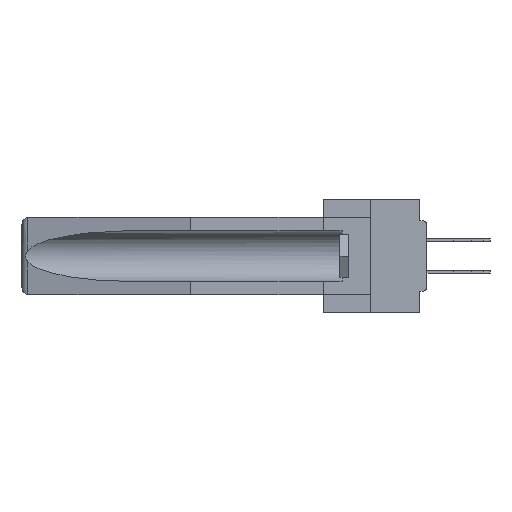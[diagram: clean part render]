
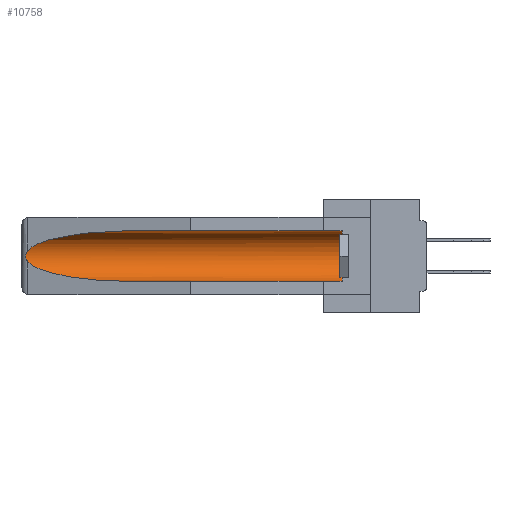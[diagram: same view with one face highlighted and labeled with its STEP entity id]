
A CAD part, left-side view. The second image highlights one B-rep face of the part: STEP entity #10758.
In plain terms, the highlighted cylindrical face has radius 2.857 mm (diameter 5.715 mm), a partial arc.
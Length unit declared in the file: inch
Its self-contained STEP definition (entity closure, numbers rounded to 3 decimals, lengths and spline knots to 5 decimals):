
#1452 = ORIENTED_EDGE ( 'NONE', *, *, #31023, .T. ) ;
#3160 = EDGE_CURVE ( 'NONE', #37127, #38480, #37272, .T. ) ;
#3463 = EDGE_CURVE ( 'NONE', #36709, #23929, #5221, .T. ) ;
#3710 = CYLINDRICAL_SURFACE ( 'NONE', #12687, 0.1125 ) ;
#5221 = LINE ( 'NONE', #6057, #36539 ) ;
#5998 = LINE ( 'NONE', #22426, #10284 ) ;
#6057 = CARTESIAN_POINT ( 'NONE',  ( 0.155, -0.30754, -0.284 ) ) ;
#6124 = VERTEX_POINT ( 'NONE', #24684 ) ;
#6145 = CARTESIAN_POINT ( 'NONE',  ( 0.26537, 1.52718, -0.14972 ) ) ;
#6793 = CARTESIAN_POINT ( 'NONE',  ( 0.26655, 1.53094, -0.18657 ) ) ;
#7048 = CARTESIAN_POINT ( 'NONE',  ( 0.26537, 1.52718, -0.14972 ) ) ;
#7515 = CARTESIAN_POINT ( 'NONE',  ( 0.25451, 1.48313, -0.24835 ) ) ;
#8026 = CARTESIAN_POINT ( 'NONE',  ( 0.155, 1.07973, -0.059 ) ) ;
#9850 = CARTESIAN_POINT ( 'NONE',  ( 0.26654, 1.53092, -0.15636 ) ) ;
#10284 = VECTOR ( 'NONE', #19735, 39.37008 ) ;
#10758 = ADVANCED_FACE ( 'NONE', ( #15102 ), #3710, .F. ) ;
#11157 = EDGE_LOOP ( 'NONE', ( #14108, #13825, #1452, #12242, #15040, #12177 ) ) ;
#12177 = ORIENTED_EDGE ( 'NONE', *, *, #22224, .T. ) ;
#12242 = ORIENTED_EDGE ( 'NONE', *, *, #3463, .F. ) ;
#12687 = AXIS2_PLACEMENT_3D ( 'NONE', #19262, #34618, #22464 ) ;
#12716 = CARTESIAN_POINT ( 'NONE',  ( 0.2675, 1.53308, -0.16763 ) ) ;
#12999 = CARTESIAN_POINT ( 'NONE',  ( 0.155, 0.126, -0.284 ) ) ;
#13016 = EDGE_CURVE ( 'NONE', #29056, #37127, #23059, .T. ) ;
#13825 = ORIENTED_EDGE ( 'NONE', *, *, #3160, .T. ) ;
#14091 = CARTESIAN_POINT ( 'NONE',  ( 0.155, 1.07973, -0.284 ) ) ;
#14108 = ORIENTED_EDGE ( 'NONE', *, *, #13016, .T. ) ;
#15003 = CARTESIAN_POINT ( 'NONE',  ( 0.155, 1.07973, -0.059 ) ) ;
#15040 = ORIENTED_EDGE ( 'NONE', *, *, #27269, .T. ) ;
#15102 = FACE_OUTER_BOUND ( 'NONE', #11157, .T. ) ;
#16002 = CARTESIAN_POINT ( 'NONE',  ( 0.2673, 1.5327, -0.16383 ) ) ;
#18591 = DIRECTION ( 'NONE',  ( 0., 0., 1. ) ) ;
#18723 = CARTESIAN_POINT ( 'NONE',  ( 0.26597, 1.5296, -0.19026 ) ) ;
#19262 = CARTESIAN_POINT ( 'NONE',  ( 0.155, -0.30754, -0.1715 ) ) ;
#19735 = DIRECTION ( 'NONE',  ( 0., 1., 0. ) ) ;
#21076 = CARTESIAN_POINT ( 'NONE',  ( 0.26537, 1.52718, -0.14972 ) ) ;
#21140 = CARTESIAN_POINT ( 'NONE',  ( 0.25451, 1.48313, -0.09465 ) ) ;
#21765 = CARTESIAN_POINT ( 'NONE',  ( 0.2675, 1.53308, -0.17534 ) ) ;
#22224 = EDGE_CURVE ( 'NONE', #6124, #29056, #5998, .T. ) ;
#22426 = CARTESIAN_POINT ( 'NONE',  ( 0.155, -0.30754, -0.059 ) ) ;
#22464 = DIRECTION ( 'NONE',  ( 0., 0., 1. ) ) ;
#23059 =( BOUNDED_CURVE ( )  B_SPLINE_CURVE ( 3, ( #15003, #33036, #21140, #6145 ),
 .UNSPECIFIED., .F., .F. ) 
 B_SPLINE_CURVE_WITH_KNOTS ( ( 4, 4 ),
 ( 4.71239, 6.08839 ),
 .UNSPECIFIED. ) 
 CURVE ( )  GEOMETRIC_REPRESENTATION_ITEM ( )  RATIONAL_B_SPLINE_CURVE ( ( 1., 0.848, 0.848, 1. ) ) 
 REPRESENTATION_ITEM ( '' )  );
#23868 = DIRECTION ( 'NONE',  ( 0., 1., 0. ) ) ;
#23929 = VERTEX_POINT ( 'NONE', #27869 ) ;
#24310 =( BOUNDED_CURVE ( )  B_SPLINE_CURVE ( 3, ( #25575, #7515, #38242, #14091 ),
 .UNSPECIFIED., .F., .F. ) 
 B_SPLINE_CURVE_WITH_KNOTS ( ( 4, 4 ),
 ( 0.1948, 1.5708 ),
 .UNSPECIFIED. ) 
 CURVE ( )  GEOMETRIC_REPRESENTATION_ITEM ( )  RATIONAL_B_SPLINE_CURVE ( ( 1., 0.848, 0.848, 1. ) ) 
 REPRESENTATION_ITEM ( '' )  );
#24684 = CARTESIAN_POINT ( 'NONE',  ( 0.155, 0.126, -0.059 ) ) ;
#25575 = CARTESIAN_POINT ( 'NONE',  ( 0.26537, 1.52718, -0.19328 ) ) ;
#27269 = EDGE_CURVE ( 'NONE', #36709, #6124, #35819, .T. ) ;
#27869 = CARTESIAN_POINT ( 'NONE',  ( 0.155, 1.07973, -0.284 ) ) ;
#29056 = VERTEX_POINT ( 'NONE', #8026 ) ;
#30701 = CARTESIAN_POINT ( 'NONE',  ( 0.155, 0.126, -0.1715 ) ) ;
#30852 = CARTESIAN_POINT ( 'NONE',  ( 0.26597, 1.52961, -0.15275 ) ) ;
#31023 = EDGE_CURVE ( 'NONE', #38480, #23929, #24310, .T. ) ;
#31125 = CARTESIAN_POINT ( 'NONE',  ( 0.26537, 1.52718, -0.19328 ) ) ;
#33036 = CARTESIAN_POINT ( 'NONE',  ( 0.21114, 1.30732, -0.059 ) ) ;
#34618 = DIRECTION ( 'NONE',  ( 0., 1., 0. ) ) ;
#35819 = CIRCLE ( 'NONE', #37713, 0.1125 ) ;
#36539 = VECTOR ( 'NONE', #23868, 39.37008 ) ;
#36709 = VERTEX_POINT ( 'NONE', #12999 ) ;
#36832 = DIRECTION ( 'NONE',  ( 0., -1., 0. ) ) ;
#36849 = CARTESIAN_POINT ( 'NONE',  ( 0.2673, 1.53269, -0.17917 ) ) ;
#37127 = VERTEX_POINT ( 'NONE', #21076 ) ;
#37272 = B_SPLINE_CURVE_WITH_KNOTS ( 'NONE', 3,
 ( #7048, #30852, #9850, #16002, #12716, #21765, #36849, #6793, #18723, #37360 ),
 .UNSPECIFIED., .F., .F.,
 ( 4, 2, 2, 2, 4 ),
 ( 0., 0.00029, 0.00058, 0.00087, 0.00117 ),
 .UNSPECIFIED. ) ;
#37360 = CARTESIAN_POINT ( 'NONE',  ( 0.26537, 1.52718, -0.19328 ) ) ;
#37713 = AXIS2_PLACEMENT_3D ( 'NONE', #30701, #36832, #18591 ) ;
#38242 = CARTESIAN_POINT ( 'NONE',  ( 0.21114, 1.30732, -0.284 ) ) ;
#38480 = VERTEX_POINT ( 'NONE', #31125 ) ;
